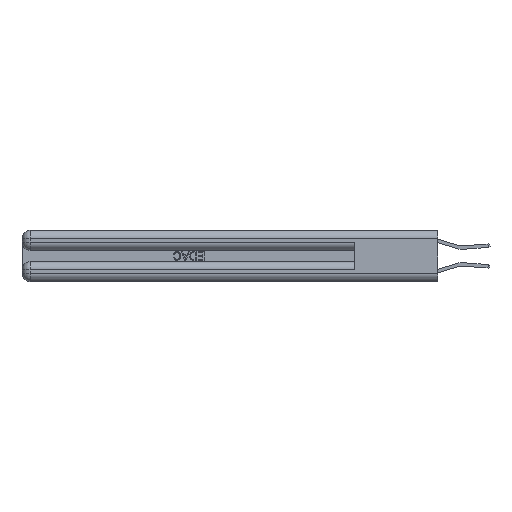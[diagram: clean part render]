
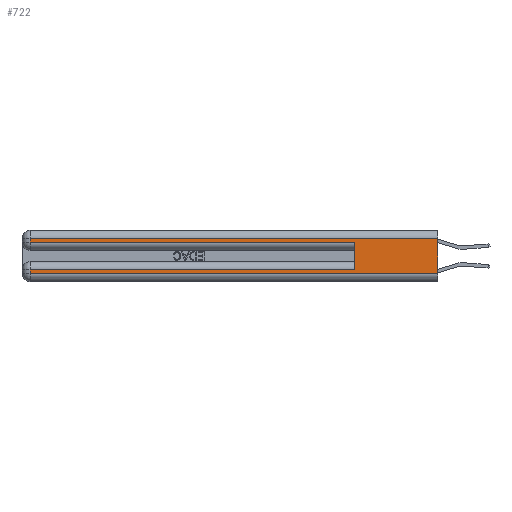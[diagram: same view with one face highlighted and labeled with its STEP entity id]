
A CAD part, left-side view. The second image highlights one B-rep face of the part: STEP entity #722.
In plain terms, the highlighted planar face has unit normal (-1, 0, 0).
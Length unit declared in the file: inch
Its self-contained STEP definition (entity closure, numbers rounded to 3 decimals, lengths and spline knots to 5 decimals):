
#149 = VERTEX_POINT ( 'NONE', #31179 ) ;
#398 = VERTEX_POINT ( 'NONE', #24899 ) ;
#463 = EDGE_CURVE ( 'NONE', #31117, #7747, #3263, .T. ) ;
#722 = ADVANCED_FACE ( 'NONE', ( #4664 ), #8926, .F. ) ;
#1251 = EDGE_CURVE ( 'NONE', #398, #149, #1572, .T. ) ;
#1331 = LINE ( 'NONE', #9908, #9391 ) ;
#1387 = VECTOR ( 'NONE', #8565, 39.37008 ) ;
#1463 = DIRECTION ( 'NONE',  ( 0., 1., 0. ) ) ;
#1572 = LINE ( 'NONE', #23628, #29510 ) ;
#1782 = ORIENTED_EDGE ( 'NONE', *, *, #7950, .T. ) ;
#1918 = DIRECTION ( 'NONE',  ( 0., 1., 0. ) ) ;
#2143 = ORIENTED_EDGE ( 'NONE', *, *, #15382, .T. ) ;
#2450 = CARTESIAN_POINT ( 'NONE',  ( 0., 2.94, 0.06 ) ) ;
#2979 = VECTOR ( 'NONE', #28065, 39.37008 ) ;
#3263 = LINE ( 'NONE', #8352, #1387 ) ;
#3857 = EDGE_LOOP ( 'NONE', ( #31669, #3942, #21791, #1782, #14402, #28038, #21849, #2143 ) ) ;
#3942 = ORIENTED_EDGE ( 'NONE', *, *, #7256, .T. ) ;
#4457 = LINE ( 'NONE', #9706, #25550 ) ;
#4664 = FACE_OUTER_BOUND ( 'NONE', #3857, .T. ) ;
#6788 = LINE ( 'NONE', #6918, #15188 ) ;
#6918 = CARTESIAN_POINT ( 'NONE',  ( 0., 2.94, 0.37 ) ) ;
#7250 = DIRECTION ( 'NONE',  ( 0., 0., -1. ) ) ;
#7256 = EDGE_CURVE ( 'NONE', #10691, #31117, #25936, .T. ) ;
#7747 = VERTEX_POINT ( 'NONE', #25974 ) ;
#7950 = EDGE_CURVE ( 'NONE', #7747, #28513, #4457, .T. ) ;
#8352 = CARTESIAN_POINT ( 'NONE',  ( 0., 2.94, 0.37 ) ) ;
#8565 = DIRECTION ( 'NONE',  ( 0., 0., -1. ) ) ;
#8903 = CARTESIAN_POINT ( 'NONE',  ( 0., 2.94, 0.31 ) ) ;
#8926 = PLANE ( 'NONE',  #12011 ) ;
#9391 = VECTOR ( 'NONE', #7250, 39.37008 ) ;
#9706 = CARTESIAN_POINT ( 'NONE',  ( 0., 0., 0.285 ) ) ;
#9908 = CARTESIAN_POINT ( 'NONE',  ( 0., 0., 0.37 ) ) ;
#10189 = LINE ( 'NONE', #10400, #21344 ) ;
#10400 = CARTESIAN_POINT ( 'NONE',  ( 0., 0.6, 0.145 ) ) ;
#10691 = VERTEX_POINT ( 'NONE', #28951 ) ;
#11391 = DIRECTION ( 'NONE',  ( 0., 0., -1. ) ) ;
#11819 = DIRECTION ( 'NONE',  ( 0., 0., -1. ) ) ;
#12011 = AXIS2_PLACEMENT_3D ( 'NONE', #28729, #31042, #11391 ) ;
#12148 = DIRECTION ( 'NONE',  ( 0., -1., 0. ) ) ;
#13526 = CARTESIAN_POINT ( 'NONE',  ( 0., 0., 0.06 ) ) ;
#14402 = ORIENTED_EDGE ( 'NONE', *, *, #16845, .F. ) ;
#14987 = VERTEX_POINT ( 'NONE', #13526 ) ;
#15188 = VECTOR ( 'NONE', #11819, 39.37008 ) ;
#15382 = EDGE_CURVE ( 'NONE', #28767, #14987, #16793, .T. ) ;
#15746 = CARTESIAN_POINT ( 'NONE',  ( 0., 0., 0.06 ) ) ;
#16399 = CARTESIAN_POINT ( 'NONE',  ( 0., 0.6, 0.285 ) ) ;
#16613 = EDGE_CURVE ( 'NONE', #149, #28767, #6788, .T. ) ;
#16793 = LINE ( 'NONE', #15746, #2979 ) ;
#16845 = EDGE_CURVE ( 'NONE', #398, #28513, #10189, .T. ) ;
#19460 = VECTOR ( 'NONE', #1918, 39.37008 ) ;
#20405 = DIRECTION ( 'NONE',  ( 0., 0., 1. ) ) ;
#21344 = VECTOR ( 'NONE', #20405, 39.37008 ) ;
#21791 = ORIENTED_EDGE ( 'NONE', *, *, #463, .T. ) ;
#21849 = ORIENTED_EDGE ( 'NONE', *, *, #16613, .T. ) ;
#21945 = EDGE_CURVE ( 'NONE', #10691, #14987, #1331, .T. ) ;
#23628 = CARTESIAN_POINT ( 'NONE',  ( 0., 0., 0.085 ) ) ;
#23986 = CARTESIAN_POINT ( 'NONE',  ( 0., 0., 0.31 ) ) ;
#24899 = CARTESIAN_POINT ( 'NONE',  ( 0., 0.6, 0.085 ) ) ;
#25550 = VECTOR ( 'NONE', #12148, 39.37008 ) ;
#25936 = LINE ( 'NONE', #23986, #19460 ) ;
#25974 = CARTESIAN_POINT ( 'NONE',  ( 0., 2.94, 0.285 ) ) ;
#28038 = ORIENTED_EDGE ( 'NONE', *, *, #1251, .T. ) ;
#28065 = DIRECTION ( 'NONE',  ( 0., -1., 0. ) ) ;
#28513 = VERTEX_POINT ( 'NONE', #16399 ) ;
#28729 = CARTESIAN_POINT ( 'NONE',  ( 0., 0., 0.37 ) ) ;
#28767 = VERTEX_POINT ( 'NONE', #2450 ) ;
#28951 = CARTESIAN_POINT ( 'NONE',  ( 0., 0., 0.31 ) ) ;
#29510 = VECTOR ( 'NONE', #1463, 39.37008 ) ;
#31042 = DIRECTION ( 'NONE',  ( 1., 0., 0. ) ) ;
#31117 = VERTEX_POINT ( 'NONE', #8903 ) ;
#31179 = CARTESIAN_POINT ( 'NONE',  ( 0., 2.94, 0.085 ) ) ;
#31669 = ORIENTED_EDGE ( 'NONE', *, *, #21945, .F. ) ;
